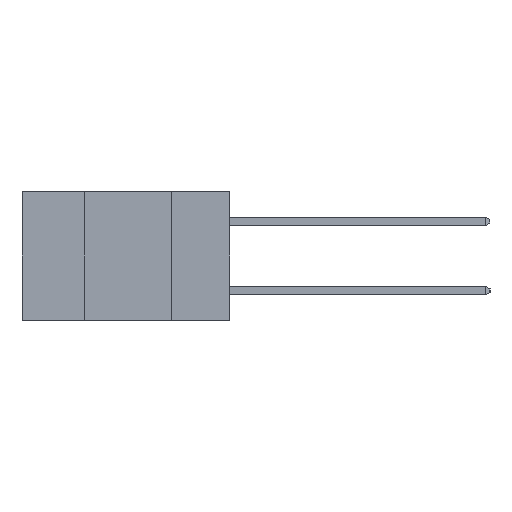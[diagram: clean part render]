
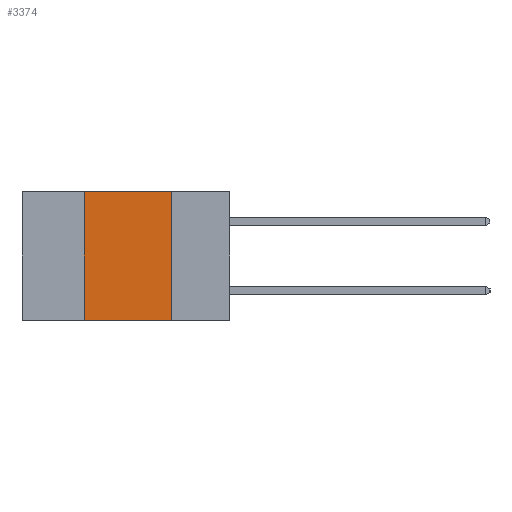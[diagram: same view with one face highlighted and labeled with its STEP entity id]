
A CAD part, left-side view. The second image highlights one B-rep face of the part: STEP entity #3374.
In plain terms, the highlighted planar face has unit normal (-1, 0, 0).
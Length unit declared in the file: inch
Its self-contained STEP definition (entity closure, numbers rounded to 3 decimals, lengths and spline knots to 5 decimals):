
#462 = CARTESIAN_POINT ( 'NONE',  ( 0., 0.6, -0.37 ) ) ;
#887 = FACE_OUTER_BOUND ( 'NONE', #21282, .T. ) ;
#2747 = EDGE_CURVE ( 'NONE', #2822, #25573, #15394, .T. ) ;
#2822 = VERTEX_POINT ( 'NONE', #17327 ) ;
#2909 = CARTESIAN_POINT ( 'NONE',  ( 0., 0.17, 0. ) ) ;
#2959 = VERTEX_POINT ( 'NONE', #4401 ) ;
#3374 = ADVANCED_FACE ( 'NONE', ( #887 ), #15633, .F. ) ;
#4401 = CARTESIAN_POINT ( 'NONE',  ( 0., 0.17, -0.37 ) ) ;
#4496 = DIRECTION ( 'NONE',  ( 0., -1., 0. ) ) ;
#5678 = CARTESIAN_POINT ( 'NONE',  ( 0., 0.42, -0.37 ) ) ;
#6137 = VECTOR ( 'NONE', #15889, 39.37008 ) ;
#7031 = VERTEX_POINT ( 'NONE', #18207 ) ;
#8497 = LINE ( 'NONE', #5678, #23780 ) ;
#8772 = ORIENTED_EDGE ( 'NONE', *, *, #2747, .F. ) ;
#10030 = VECTOR ( 'NONE', #24467, 39.37008 ) ;
#10674 = AXIS2_PLACEMENT_3D ( 'NONE', #18355, #18408, #18435 ) ;
#11009 = ORIENTED_EDGE ( 'NONE', *, *, #12692, .F. ) ;
#11518 = EDGE_CURVE ( 'NONE', #7031, #2959, #24639, .T. ) ;
#12692 = EDGE_CURVE ( 'NONE', #25573, #2959, #22084, .T. ) ;
#13769 = DIRECTION ( 'NONE',  ( 0., 0., 1. ) ) ;
#15394 = LINE ( 'NONE', #15486, #10030 ) ;
#15486 = CARTESIAN_POINT ( 'NONE',  ( 0., 0.6, 0. ) ) ;
#15633 = PLANE ( 'NONE',  #10674 ) ;
#15889 = DIRECTION ( 'NONE',  ( 0., 0., -1. ) ) ;
#17327 = CARTESIAN_POINT ( 'NONE',  ( 0., 0.42, 0. ) ) ;
#17893 = CARTESIAN_POINT ( 'NONE',  ( 0., 0.17, -0.37 ) ) ;
#18207 = CARTESIAN_POINT ( 'NONE',  ( 0., 0.42, -0.37 ) ) ;
#18355 = CARTESIAN_POINT ( 'NONE',  ( 0., 0.6, 0. ) ) ;
#18408 = DIRECTION ( 'NONE',  ( 1., 0., 0. ) ) ;
#18435 = DIRECTION ( 'NONE',  ( 0., 0., -1. ) ) ;
#19411 = VECTOR ( 'NONE', #4496, 39.37008 ) ;
#20024 = EDGE_CURVE ( 'NONE', #7031, #2822, #8497, .T. ) ;
#20035 = ORIENTED_EDGE ( 'NONE', *, *, #20024, .F. ) ;
#21282 = EDGE_LOOP ( 'NONE', ( #11009, #8772, #20035, #25263 ) ) ;
#22084 = LINE ( 'NONE', #17893, #6137 ) ;
#23780 = VECTOR ( 'NONE', #13769, 39.37008 ) ;
#24467 = DIRECTION ( 'NONE',  ( 0., -1., 0. ) ) ;
#24639 = LINE ( 'NONE', #462, #19411 ) ;
#25263 = ORIENTED_EDGE ( 'NONE', *, *, #11518, .T. ) ;
#25573 = VERTEX_POINT ( 'NONE', #2909 ) ;
